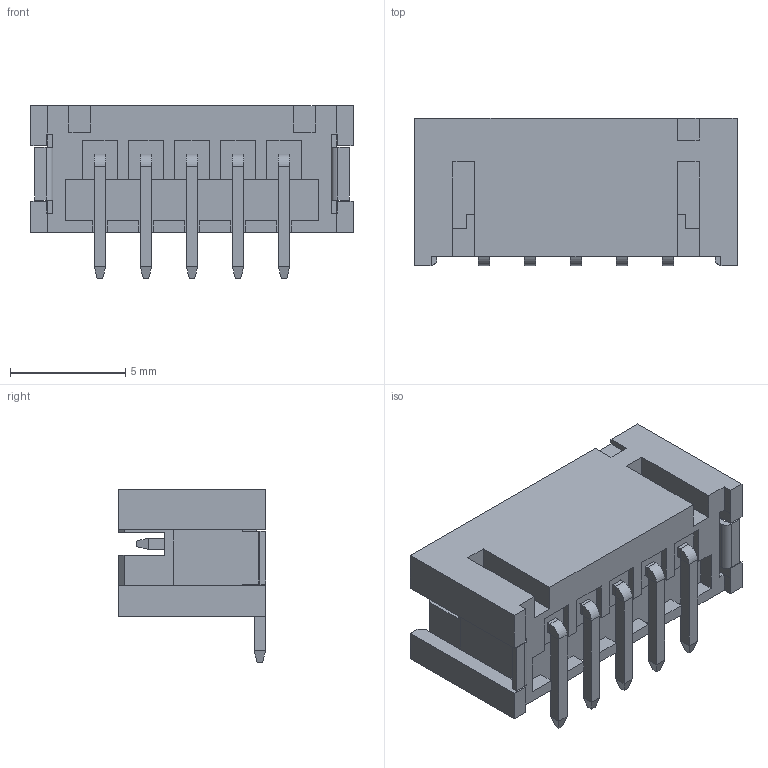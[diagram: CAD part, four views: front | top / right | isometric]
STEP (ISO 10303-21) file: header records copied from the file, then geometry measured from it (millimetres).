
FILE_DESCRIPTION (( 'STEP AP203' ), '1' );
FILE_NAME ('140-505-417-011.STEP', '2020-03-31T20:02:29', ( '' ), ( '' ), 'SwSTEP 2.0', 'SolidWorks 2016', '' );
FILE_SCHEMA (( 'CONFIG_CONTROL_DESIGN' ));
Length unit declared in the file: millimetre
Products named in the file (4): V SMT Pad; V SMT Contact; 140-505-417-011; V SMT Housing_505
Assembly tree (8 placements, depth 2):
  140-505-417-011
    V SMT Housing_505
    V SMT Contact  x5
    V SMT Pad  x2
Bounding box: 14 x 6.4 x 7.5 mm (x, y, z)
Volume: 222.5 mm3; surface area: 795.3 mm2
Topology: 8 solids, 8 shells, 290 faces, 744 edges, 466 vertices
Faces by surface type: plane 276, cylinder 14
Entity records: 6538 total; most frequent: CARTESIAN_POINT 1077, ORIENTED_EDGE 1064, DIRECTION 938, EDGE_CURVE 532, VECTOR 524, LINE 524, VERTEX_POINT 346, AXIS2_PLACEMENT_3D 207
